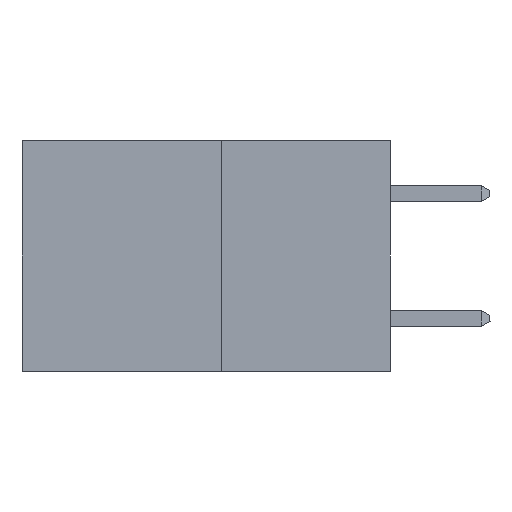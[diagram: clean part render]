
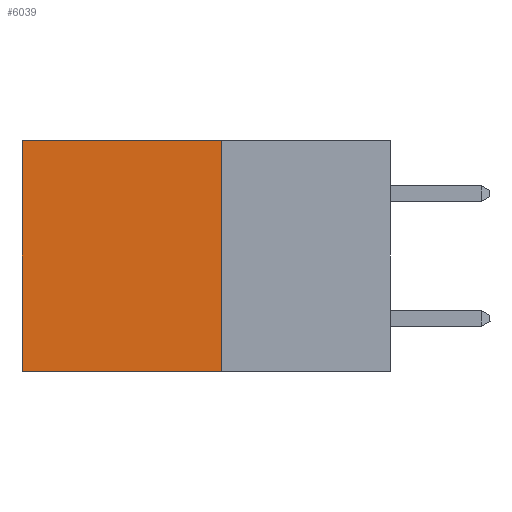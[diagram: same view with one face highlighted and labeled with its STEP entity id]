
A CAD part, left-side view. The second image highlights one B-rep face of the part: STEP entity #6039.
In plain terms, the highlighted planar face has unit normal (-1, 0, 0).
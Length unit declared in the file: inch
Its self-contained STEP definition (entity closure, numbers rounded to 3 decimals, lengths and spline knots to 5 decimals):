
#176 = ORIENTED_EDGE ( 'NONE', *, *, #3650, .T. ) ;
#296 = VECTOR ( 'NONE', #4262, 39.37008 ) ;
#978 = EDGE_CURVE ( 'NONE', #15141, #8198, #14175, .T. ) ;
#1952 = ORIENTED_EDGE ( 'NONE', *, *, #8897, .T. ) ;
#1965 = CARTESIAN_POINT ( 'NONE',  ( 0.277, 0.27, -0.37 ) ) ;
#2223 = CARTESIAN_POINT ( 'NONE',  ( 0.277, 0.27, 0. ) ) ;
#2525 = CARTESIAN_POINT ( 'NONE',  ( 0.277, 0.27, -0.37 ) ) ;
#3339 = ORIENTED_EDGE ( 'NONE', *, *, #978, .F. ) ;
#3650 = EDGE_CURVE ( 'NONE', #15141, #19034, #18945, .T. ) ;
#4262 = DIRECTION ( 'NONE',  ( 0., 0., -1. ) ) ;
#4570 = CARTESIAN_POINT ( 'NONE',  ( 0.277, 0.27, -0.37 ) ) ;
#4738 = LINE ( 'NONE', #9267, #296 ) ;
#5273 = PLANE ( 'NONE',  #11068 ) ;
#6039 = ADVANCED_FACE ( 'NONE', ( #7497 ), #5273, .F. ) ;
#7497 = FACE_OUTER_BOUND ( 'NONE', #13709, .T. ) ;
#8198 = VERTEX_POINT ( 'NONE', #20713 ) ;
#8666 = DIRECTION ( 'NONE',  ( 0., 0., -1. ) ) ;
#8897 = EDGE_CURVE ( 'NONE', #19034, #15585, #4738, .T. ) ;
#9267 = CARTESIAN_POINT ( 'NONE',  ( 0.277, 0.59, -0.37 ) ) ;
#9275 = VECTOR ( 'NONE', #9548, 39.37008 ) ;
#9492 = CARTESIAN_POINT ( 'NONE',  ( 0.277, 0.59, 0. ) ) ;
#9548 = DIRECTION ( 'NONE',  ( 0., 0., -1. ) ) ;
#9887 = CARTESIAN_POINT ( 'NONE',  ( 0.277, 0.59, -0.37 ) ) ;
#11068 = AXIS2_PLACEMENT_3D ( 'NONE', #1965, #18529, #8666 ) ;
#11298 = CARTESIAN_POINT ( 'NONE',  ( 0.277, 0.27, 0. ) ) ;
#12734 = LINE ( 'NONE', #2525, #17080 ) ;
#13709 = EDGE_LOOP ( 'NONE', ( #1952, #13943, #3339, #176 ) ) ;
#13943 = ORIENTED_EDGE ( 'NONE', *, *, #19578, .F. ) ;
#14175 = LINE ( 'NONE', #4570, #9275 ) ;
#14675 = DIRECTION ( 'NONE',  ( 0., 1., 0. ) ) ;
#15141 = VERTEX_POINT ( 'NONE', #2223 ) ;
#15585 = VERTEX_POINT ( 'NONE', #9887 ) ;
#15797 = DIRECTION ( 'NONE',  ( 0., 1., 0. ) ) ;
#17080 = VECTOR ( 'NONE', #15797, 39.37008 ) ;
#18417 = VECTOR ( 'NONE', #14675, 39.37008 ) ;
#18529 = DIRECTION ( 'NONE',  ( 1., 0., 0. ) ) ;
#18945 = LINE ( 'NONE', #11298, #18417 ) ;
#19034 = VERTEX_POINT ( 'NONE', #9492 ) ;
#19578 = EDGE_CURVE ( 'NONE', #8198, #15585, #12734, .T. ) ;
#20713 = CARTESIAN_POINT ( 'NONE',  ( 0.277, 0.27, -0.37 ) ) ;
